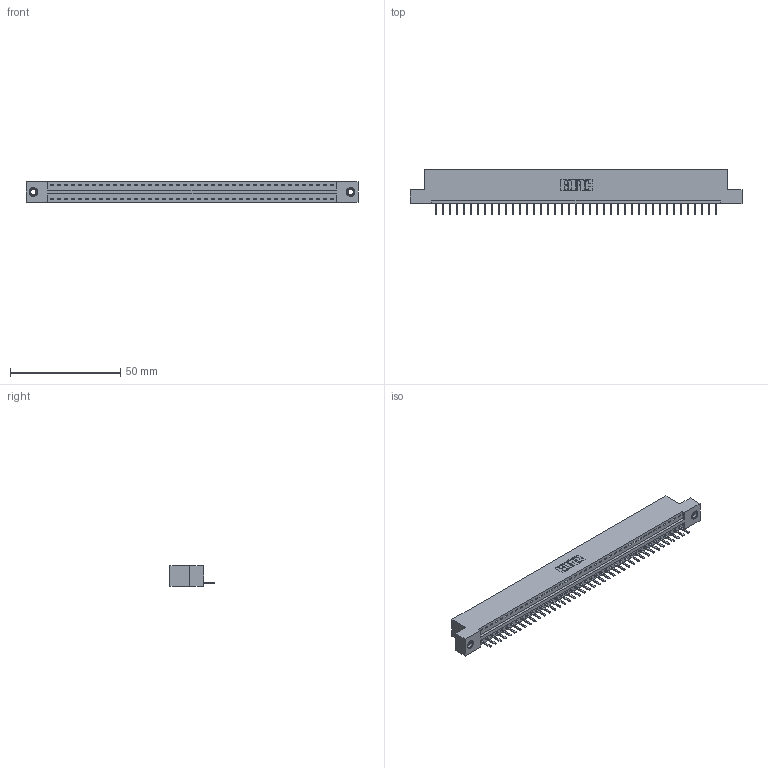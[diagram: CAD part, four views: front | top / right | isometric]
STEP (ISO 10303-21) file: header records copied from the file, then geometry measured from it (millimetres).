
FILE_DESCRIPTION (( 'STEP AP203' ), '1' );
FILE_NAME ('346-041-520-107.STEP', '2022-05-07T11:05:31', ( '' ), ( '' ), 'SwSTEP 2.0', 'SolidWorks 2020', '' );
FILE_SCHEMA (( 'CONFIG_CONTROL_DESIGN' ));
Length unit declared in the file: inch
Products named in the file (4): 345-250-001_345-250-005-103; 346-041-520-107; 345-292-001_345-293-120; 346 Part_Flush Mounting Lugs - 0.156 Dia-TI
Assembly tree (44 placements, depth 2):
  346-041-520-107
    346 Part_Flush Mounting Lugs - 0.156 Dia-TI
    345-292-001_345-293-120  x41
    345-250-001_345-250-005-103  x2
Bounding box: 150.75 x 20.02 x 9.4 mm (x, y, z)
Volume: 14291.7 mm3; surface area: 17492.9 mm2
Topology: 44 solids, 44 shells, 2724 faces, 8009 edges, 5222 vertices
Faces by surface type: plane 1830, cylinder 878, cone 12, torus 4
Entity records: 26880 total; most frequent: CARTESIAN_POINT 4602, ORIENTED_EDGE 4558, DIRECTION 4075, EDGE_CURVE 2279, LINE 1959, VECTOR 1959, VERTEX_POINT 1512, AXIS2_PLACEMENT_3D 1058
